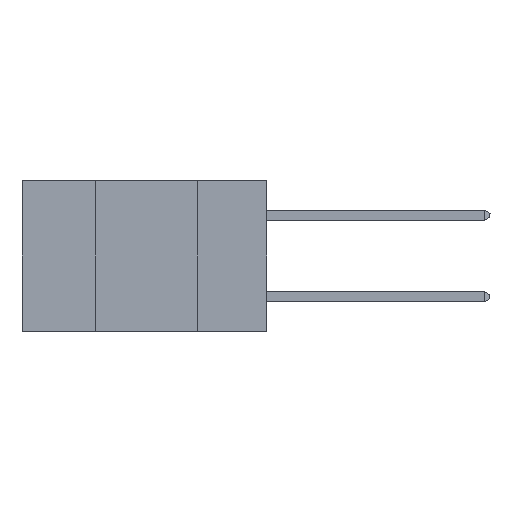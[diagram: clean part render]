
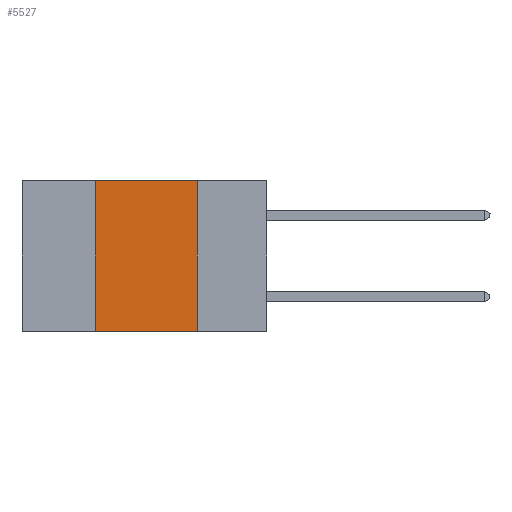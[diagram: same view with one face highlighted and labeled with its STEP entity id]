
A CAD part, left-side view. The second image highlights one B-rep face of the part: STEP entity #5527.
In plain terms, the highlighted planar face has unit normal (-1, 0, 0).
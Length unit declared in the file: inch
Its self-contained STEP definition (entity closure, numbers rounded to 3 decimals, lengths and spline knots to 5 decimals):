
#196 = CARTESIAN_POINT ( 'NONE',  ( 0., 0.42, -0.37 ) ) ;
#979 = EDGE_CURVE ( 'NONE', #17370, #27367, #7254, .T. ) ;
#3137 = ORIENTED_EDGE ( 'NONE', *, *, #979, .F. ) ;
#3452 = EDGE_LOOP ( 'NONE', ( #3137, #16206, #19164, #26086 ) ) ;
#4536 = CARTESIAN_POINT ( 'NONE',  ( 0., 0.42, 0. ) ) ;
#4900 = DIRECTION ( 'NONE',  ( 0., -1., 0. ) ) ;
#5398 = EDGE_CURVE ( 'NONE', #18984, #17370, #12251, .T. ) ;
#5527 = ADVANCED_FACE ( 'NONE', ( #6253 ), #14802, .F. ) ;
#6253 = FACE_OUTER_BOUND ( 'NONE', #3452, .T. ) ;
#7254 = LINE ( 'NONE', #27379, #8527 ) ;
#7427 = LINE ( 'NONE', #12063, #7435 ) ;
#7435 = VECTOR ( 'NONE', #21202, 39.37008 ) ;
#8527 = VECTOR ( 'NONE', #15957, 39.37008 ) ;
#8806 = VECTOR ( 'NONE', #20856, 39.37008 ) ;
#11961 = CARTESIAN_POINT ( 'NONE',  ( 0., 0.42, 0. ) ) ;
#12063 = CARTESIAN_POINT ( 'NONE',  ( 0., 0.6, -0.37 ) ) ;
#12251 = LINE ( 'NONE', #18985, #23929 ) ;
#12712 = EDGE_CURVE ( 'NONE', #20761, #27367, #7427, .T. ) ;
#12995 = CARTESIAN_POINT ( 'NONE',  ( 0., 0.6, 0. ) ) ;
#14802 = PLANE ( 'NONE',  #20594 ) ;
#15957 = DIRECTION ( 'NONE',  ( 0., 0., -1. ) ) ;
#16206 = ORIENTED_EDGE ( 'NONE', *, *, #5398, .F. ) ;
#16434 = EDGE_CURVE ( 'NONE', #20761, #18984, #27798, .T. ) ;
#17370 = VERTEX_POINT ( 'NONE', #20362 ) ;
#18984 = VERTEX_POINT ( 'NONE', #11961 ) ;
#18985 = CARTESIAN_POINT ( 'NONE',  ( 0., 0.6, 0. ) ) ;
#19164 = ORIENTED_EDGE ( 'NONE', *, *, #16434, .F. ) ;
#19434 = DIRECTION ( 'NONE',  ( 1., 0., 0. ) ) ;
#20362 = CARTESIAN_POINT ( 'NONE',  ( 0., 0.17, 0. ) ) ;
#20594 = AXIS2_PLACEMENT_3D ( 'NONE', #12995, #19434, #21829 ) ;
#20761 = VERTEX_POINT ( 'NONE', #196 ) ;
#20856 = DIRECTION ( 'NONE',  ( 0., 0., 1. ) ) ;
#21202 = DIRECTION ( 'NONE',  ( 0., -1., 0. ) ) ;
#21829 = DIRECTION ( 'NONE',  ( 0., 0., -1. ) ) ;
#23929 = VECTOR ( 'NONE', #4900, 39.37008 ) ;
#26086 = ORIENTED_EDGE ( 'NONE', *, *, #12712, .T. ) ;
#27314 = CARTESIAN_POINT ( 'NONE',  ( 0., 0.17, -0.37 ) ) ;
#27367 = VERTEX_POINT ( 'NONE', #27314 ) ;
#27379 = CARTESIAN_POINT ( 'NONE',  ( 0., 0.17, 0. ) ) ;
#27798 = LINE ( 'NONE', #4536, #8806 ) ;
